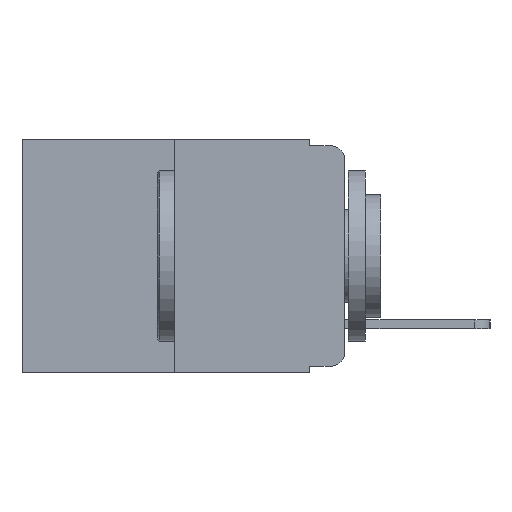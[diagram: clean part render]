
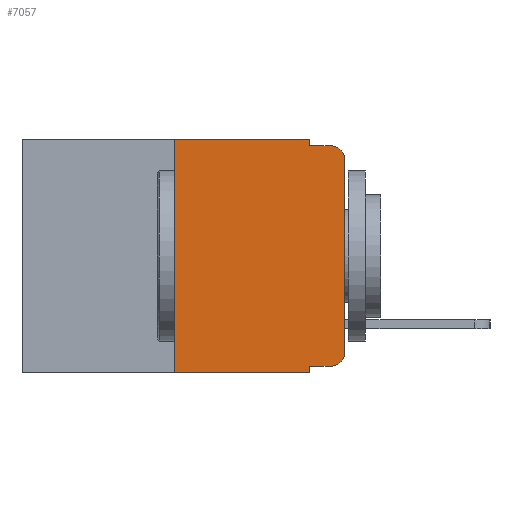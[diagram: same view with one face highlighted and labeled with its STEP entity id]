
A CAD part, left-side view. The second image highlights one B-rep face of the part: STEP entity #7057.
In plain terms, the highlighted planar face has unit normal (-1, 0, 0).
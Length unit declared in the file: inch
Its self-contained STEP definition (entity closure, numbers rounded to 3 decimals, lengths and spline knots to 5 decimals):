
#135 = ORIENTED_EDGE ( 'NONE', *, *, #3885, .F. ) ;
#165 = ORIENTED_EDGE ( 'NONE', *, *, #9334, .F. ) ;
#218 = ORIENTED_EDGE ( 'NONE', *, *, #6657, .F. ) ;
#274 = ORIENTED_EDGE ( 'NONE', *, *, #8502, .F. ) ;
#387 = EDGE_CURVE ( 'NONE', #1037, #967, #7949, .T. ) ;
#391 = VERTEX_POINT ( 'NONE', #10071 ) ;
#395 = ORIENTED_EDGE ( 'NONE', *, *, #10230, .T. ) ;
#412 = VERTEX_POINT ( 'NONE', #8260 ) ;
#545 = ORIENTED_EDGE ( 'NONE', *, *, #11369, .T. ) ;
#611 = CARTESIAN_POINT ( 'NONE',  ( 0., 0.051, 0. ) ) ;
#727 = DIRECTION ( 'NONE',  ( 0., -1., 0. ) ) ;
#768 = CARTESIAN_POINT ( 'NONE',  ( 0., 0., -0.313 ) ) ;
#946 = CARTESIAN_POINT ( 'NONE',  ( 0., 0.25, 0. ) ) ;
#967 = VERTEX_POINT ( 'NONE', #11481 ) ;
#1037 = VERTEX_POINT ( 'NONE', #3506 ) ;
#1135 = EDGE_CURVE ( 'NONE', #412, #6294, #8992, .T. ) ;
#1153 = AXIS2_PLACEMENT_3D ( 'NONE', #10344, #7830, #1691 ) ;
#1207 = VERTEX_POINT ( 'NONE', #11812 ) ;
#1295 = CARTESIAN_POINT ( 'NONE',  ( 0., 0., -0.03 ) ) ;
#1303 = EDGE_LOOP ( 'NONE', ( #545, #395, #274, #218, #165, #135, #7639, #11942, #5413, #4168 ) ) ;
#1309 = LINE ( 'NONE', #946, #5529 ) ;
#1335 = VERTEX_POINT ( 'NONE', #6093 ) ;
#1691 = DIRECTION ( 'NONE',  ( 0., 0., -1. ) ) ;
#2285 = AXIS2_PLACEMENT_3D ( 'NONE', #11188, #5838, #12056 ) ;
#2463 = DIRECTION ( 'NONE',  ( 0., 0., -1. ) ) ;
#2486 = EDGE_CURVE ( 'NONE', #1037, #6294, #7916, .T. ) ;
#2773 = DIRECTION ( 'NONE',  ( 0., 0., 1. ) ) ;
#3097 = LINE ( 'NONE', #5946, #8657 ) ;
#3506 = CARTESIAN_POINT ( 'NONE',  ( 0., 0.051, -0.333 ) ) ;
#3885 = EDGE_CURVE ( 'NONE', #412, #1207, #1309, .T. ) ;
#3914 = VECTOR ( 'NONE', #10322, 39.37008 ) ;
#3920 = CARTESIAN_POINT ( 'NONE',  ( 0., 0.473, -0.343 ) ) ;
#4168 = ORIENTED_EDGE ( 'NONE', *, *, #12160, .T. ) ;
#4449 = LINE ( 'NONE', #10526, #11776 ) ;
#4474 = FACE_OUTER_BOUND ( 'NONE', #1303, .T. ) ;
#4653 = VERTEX_POINT ( 'NONE', #1295 ) ;
#4764 = PLANE ( 'NONE',  #1153 ) ;
#4923 = CARTESIAN_POINT ( 'NONE',  ( 0., 0.02, -0.03 ) ) ;
#5295 = VECTOR ( 'NONE', #8286, 39.37008 ) ;
#5413 = ORIENTED_EDGE ( 'NONE', *, *, #387, .T. ) ;
#5529 = VECTOR ( 'NONE', #9024, 39.37008 ) ;
#5592 = VERTEX_POINT ( 'NONE', #768 ) ;
#5838 = DIRECTION ( 'NONE',  ( -1., 0., 0. ) ) ;
#5916 = CIRCLE ( 'NONE', #10691, 0.02 ) ;
#5946 = CARTESIAN_POINT ( 'NONE',  ( 0., 0., 0. ) ) ;
#5999 = DIRECTION ( 'NONE',  ( 0., 0., -1. ) ) ;
#6025 = CIRCLE ( 'NONE', #2285, 0.02 ) ;
#6093 = CARTESIAN_POINT ( 'NONE',  ( 0., 0.051, -0.01 ) ) ;
#6294 = VERTEX_POINT ( 'NONE', #9631 ) ;
#6406 = DIRECTION ( 'NONE',  ( 0., -1., 0. ) ) ;
#6480 = CARTESIAN_POINT ( 'NONE',  ( 0., 0.051, -0.333 ) ) ;
#6569 = VECTOR ( 'NONE', #6406, 39.37008 ) ;
#6657 = EDGE_CURVE ( 'NONE', #391, #1335, #6969, .T. ) ;
#6969 = LINE ( 'NONE', #611, #3914 ) ;
#7057 = ADVANCED_FACE ( 'NONE', ( #4474 ), #4764, .F. ) ;
#7309 = CARTESIAN_POINT ( 'NONE',  ( 0., 0.051, 0. ) ) ;
#7639 = ORIENTED_EDGE ( 'NONE', *, *, #1135, .T. ) ;
#7830 = DIRECTION ( 'NONE',  ( 1., 0., 0. ) ) ;
#7916 = LINE ( 'NONE', #7309, #10168 ) ;
#7949 = LINE ( 'NONE', #6480, #5295 ) ;
#8008 = DIRECTION ( 'NONE',  ( 0., -1., 0. ) ) ;
#8260 = CARTESIAN_POINT ( 'NONE',  ( 0., 0.25, -0.343 ) ) ;
#8286 = DIRECTION ( 'NONE',  ( 0., -1., 0. ) ) ;
#8502 = EDGE_CURVE ( 'NONE', #1335, #10092, #4449, .T. ) ;
#8657 = VECTOR ( 'NONE', #2773, 39.37008 ) ;
#8992 = LINE ( 'NONE', #3920, #6569 ) ;
#9024 = DIRECTION ( 'NONE',  ( 0., 0., 1. ) ) ;
#9334 = EDGE_CURVE ( 'NONE', #1207, #391, #9894, .T. ) ;
#9631 = CARTESIAN_POINT ( 'NONE',  ( 0., 0.051, -0.343 ) ) ;
#9894 = LINE ( 'NONE', #10402, #11904 ) ;
#10071 = CARTESIAN_POINT ( 'NONE',  ( 0., 0.051, 0. ) ) ;
#10092 = VERTEX_POINT ( 'NONE', #11964 ) ;
#10168 = VECTOR ( 'NONE', #2463, 39.37008 ) ;
#10230 = EDGE_CURVE ( 'NONE', #4653, #10092, #5916, .T. ) ;
#10322 = DIRECTION ( 'NONE',  ( 0., 0., -1. ) ) ;
#10344 = CARTESIAN_POINT ( 'NONE',  ( 0., 0.473, 0. ) ) ;
#10402 = CARTESIAN_POINT ( 'NONE',  ( 0., 0.473, 0. ) ) ;
#10526 = CARTESIAN_POINT ( 'NONE',  ( 0., 0.051, -0.01 ) ) ;
#10691 = AXIS2_PLACEMENT_3D ( 'NONE', #4923, #11325, #5999 ) ;
#11188 = CARTESIAN_POINT ( 'NONE',  ( 0., 0.02, -0.313 ) ) ;
#11325 = DIRECTION ( 'NONE',  ( -1., 0., 0. ) ) ;
#11369 = EDGE_CURVE ( 'NONE', #5592, #4653, #3097, .T. ) ;
#11481 = CARTESIAN_POINT ( 'NONE',  ( 0., 0.02, -0.333 ) ) ;
#11776 = VECTOR ( 'NONE', #8008, 39.37008 ) ;
#11812 = CARTESIAN_POINT ( 'NONE',  ( 0., 0.25, 0. ) ) ;
#11904 = VECTOR ( 'NONE', #727, 39.37008 ) ;
#11942 = ORIENTED_EDGE ( 'NONE', *, *, #2486, .F. ) ;
#11964 = CARTESIAN_POINT ( 'NONE',  ( 0., 0.02, -0.01 ) ) ;
#12056 = DIRECTION ( 'NONE',  ( 0., 0., -1. ) ) ;
#12160 = EDGE_CURVE ( 'NONE', #967, #5592, #6025, .T. ) ;
